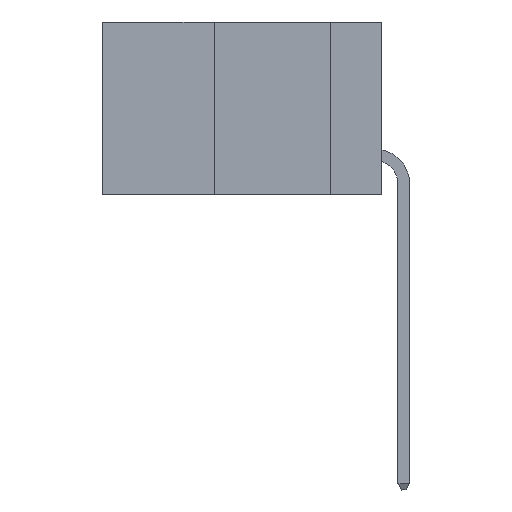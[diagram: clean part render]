
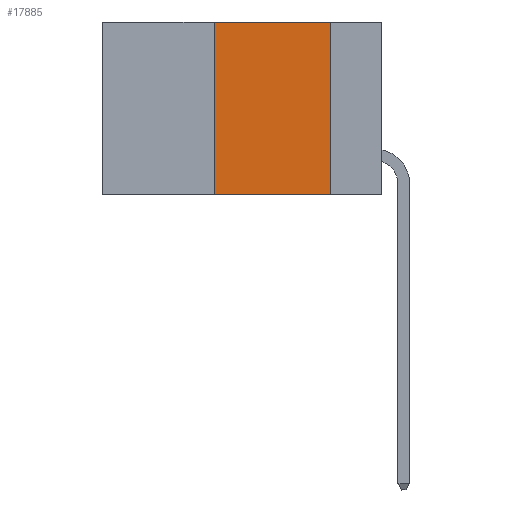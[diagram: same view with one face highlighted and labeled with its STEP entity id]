
A CAD part, left-side view. The second image highlights one B-rep face of the part: STEP entity #17885.
In plain terms, the highlighted planar face has unit normal (-1, 0, 0).
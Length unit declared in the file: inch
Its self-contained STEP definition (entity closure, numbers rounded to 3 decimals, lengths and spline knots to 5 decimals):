
#1712 = EDGE_CURVE ( 'NONE', #11967, #46711, #26788, .T. ) ;
#2717 = VECTOR ( 'NONE', #15578, 39.37008 ) ;
#4117 = ORIENTED_EDGE ( 'NONE', *, *, #34583, .F. ) ;
#5035 = CARTESIAN_POINT ( 'NONE',  ( 0., 0.6, -0.37 ) ) ;
#5591 = CARTESIAN_POINT ( 'NONE',  ( 0., 0.11, 0. ) ) ;
#11339 = CARTESIAN_POINT ( 'NONE',  ( 0., 0.6, 0. ) ) ;
#11967 = VERTEX_POINT ( 'NONE', #14808 ) ;
#13893 = DIRECTION ( 'NONE',  ( 0., -1., 0. ) ) ;
#14771 = ORIENTED_EDGE ( 'NONE', *, *, #23017, .F. ) ;
#14808 = CARTESIAN_POINT ( 'NONE',  ( 0., 0.36, -0.37 ) ) ;
#15578 = DIRECTION ( 'NONE',  ( 0., -1., 0. ) ) ;
#16771 = FACE_OUTER_BOUND ( 'NONE', #18045, .T. ) ;
#17827 = DIRECTION ( 'NONE',  ( 0., 0., 1. ) ) ;
#17885 = ADVANCED_FACE ( 'NONE', ( #16771 ), #26010, .F. ) ;
#18045 = EDGE_LOOP ( 'NONE', ( #14771, #4117, #37709, #24897 ) ) ;
#18439 = CARTESIAN_POINT ( 'NONE',  ( 0., 0.11, -0.37 ) ) ;
#19087 = VECTOR ( 'NONE', #32383, 39.37008 ) ;
#22248 = VERTEX_POINT ( 'NONE', #34493 ) ;
#23017 = EDGE_CURVE ( 'NONE', #22248, #32395, #34355, .T. ) ;
#24897 = ORIENTED_EDGE ( 'NONE', *, *, #45063, .T. ) ;
#26010 = PLANE ( 'NONE',  #35562 ) ;
#26468 = DIRECTION ( 'NONE',  ( 0., 0., -1. ) ) ;
#26788 = LINE ( 'NONE', #33254, #29777 ) ;
#27298 = LINE ( 'NONE', #29019, #36689 ) ;
#29019 = CARTESIAN_POINT ( 'NONE',  ( 0., 0.6, 0. ) ) ;
#29777 = VECTOR ( 'NONE', #17827, 39.37008 ) ;
#30097 = DIRECTION ( 'NONE',  ( 1., 0., 0. ) ) ;
#32383 = DIRECTION ( 'NONE',  ( 0., 0., -1. ) ) ;
#32395 = VERTEX_POINT ( 'NONE', #18439 ) ;
#33254 = CARTESIAN_POINT ( 'NONE',  ( 0., 0.36, 0. ) ) ;
#34355 = LINE ( 'NONE', #5591, #19087 ) ;
#34493 = CARTESIAN_POINT ( 'NONE',  ( 0., 0.11, 0. ) ) ;
#34583 = EDGE_CURVE ( 'NONE', #46711, #22248, #27298, .T. ) ;
#35562 = AXIS2_PLACEMENT_3D ( 'NONE', #11339, #30097, #26468 ) ;
#36689 = VECTOR ( 'NONE', #13893, 39.37008 ) ;
#36796 = LINE ( 'NONE', #5035, #2717 ) ;
#37563 = CARTESIAN_POINT ( 'NONE',  ( 0., 0.36, 0. ) ) ;
#37709 = ORIENTED_EDGE ( 'NONE', *, *, #1712, .F. ) ;
#45063 = EDGE_CURVE ( 'NONE', #11967, #32395, #36796, .T. ) ;
#46711 = VERTEX_POINT ( 'NONE', #37563 ) ;
